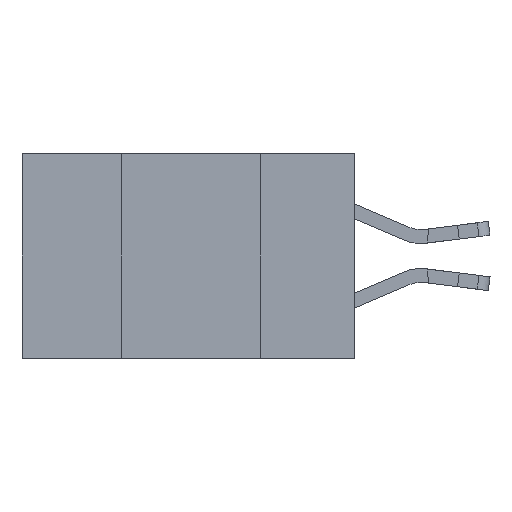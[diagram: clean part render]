
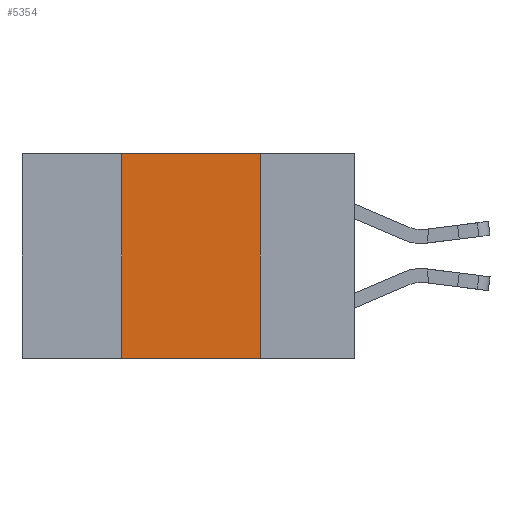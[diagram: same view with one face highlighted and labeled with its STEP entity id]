
A CAD part, left-side view. The second image highlights one B-rep face of the part: STEP entity #5354.
In plain terms, the highlighted planar face has unit normal (-1, 0, 0).
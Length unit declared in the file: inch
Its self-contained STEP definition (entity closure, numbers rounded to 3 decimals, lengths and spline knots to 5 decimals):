
#236 = DIRECTION ( 'NONE',  ( 0., 0., 1. ) ) ;
#662 = ORIENTED_EDGE ( 'NONE', *, *, #6649, .T. ) ;
#767 = AXIS2_PLACEMENT_3D ( 'NONE', #5530, #13043, #15669 ) ;
#1278 = VECTOR ( 'NONE', #9436, 39.37008 ) ;
#1502 = CARTESIAN_POINT ( 'NONE',  ( 0., 0.6, -0.37 ) ) ;
#1608 = CARTESIAN_POINT ( 'NONE',  ( 0., 0.42, -0.37 ) ) ;
#3108 = CARTESIAN_POINT ( 'NONE',  ( 0., 0.42, 0. ) ) ;
#3784 = EDGE_LOOP ( 'NONE', ( #11205, #11978, #7156, #662 ) ) ;
#3932 = VERTEX_POINT ( 'NONE', #12146 ) ;
#4048 = EDGE_CURVE ( 'NONE', #12193, #3932, #5817, .T. ) ;
#5088 = DIRECTION ( 'NONE',  ( 0., -1., 0. ) ) ;
#5354 = ADVANCED_FACE ( 'NONE', ( #13427 ), #5633, .F. ) ;
#5408 = CARTESIAN_POINT ( 'NONE',  ( 0., 0.17, 0. ) ) ;
#5530 = CARTESIAN_POINT ( 'NONE',  ( 0., 0.6, 0. ) ) ;
#5633 = PLANE ( 'NONE',  #767 ) ;
#5817 = LINE ( 'NONE', #8061, #1278 ) ;
#6649 = EDGE_CURVE ( 'NONE', #8103, #10645, #10442, .T. ) ;
#7156 = ORIENTED_EDGE ( 'NONE', *, *, #12871, .F. ) ;
#8061 = CARTESIAN_POINT ( 'NONE',  ( 0., 0.6, 0. ) ) ;
#8103 = VERTEX_POINT ( 'NONE', #1608 ) ;
#8498 = LINE ( 'NONE', #5408, #15557 ) ;
#9436 = DIRECTION ( 'NONE',  ( 0., -1., 0. ) ) ;
#9890 = VECTOR ( 'NONE', #236, 39.37008 ) ;
#10442 = LINE ( 'NONE', #1502, #14734 ) ;
#10645 = VERTEX_POINT ( 'NONE', #12831 ) ;
#11205 = ORIENTED_EDGE ( 'NONE', *, *, #13021, .F. ) ;
#11614 = CARTESIAN_POINT ( 'NONE',  ( 0., 0.42, 0. ) ) ;
#11715 = DIRECTION ( 'NONE',  ( 0., 0., -1. ) ) ;
#11978 = ORIENTED_EDGE ( 'NONE', *, *, #4048, .F. ) ;
#12146 = CARTESIAN_POINT ( 'NONE',  ( 0., 0.17, 0. ) ) ;
#12193 = VERTEX_POINT ( 'NONE', #3108 ) ;
#12831 = CARTESIAN_POINT ( 'NONE',  ( 0., 0.17, -0.37 ) ) ;
#12871 = EDGE_CURVE ( 'NONE', #8103, #12193, #15763, .T. ) ;
#13021 = EDGE_CURVE ( 'NONE', #3932, #10645, #8498, .T. ) ;
#13043 = DIRECTION ( 'NONE',  ( 1., 0., 0. ) ) ;
#13427 = FACE_OUTER_BOUND ( 'NONE', #3784, .T. ) ;
#14734 = VECTOR ( 'NONE', #5088, 39.37008 ) ;
#15557 = VECTOR ( 'NONE', #11715, 39.37008 ) ;
#15669 = DIRECTION ( 'NONE',  ( 0., 0., -1. ) ) ;
#15763 = LINE ( 'NONE', #11614, #9890 ) ;
